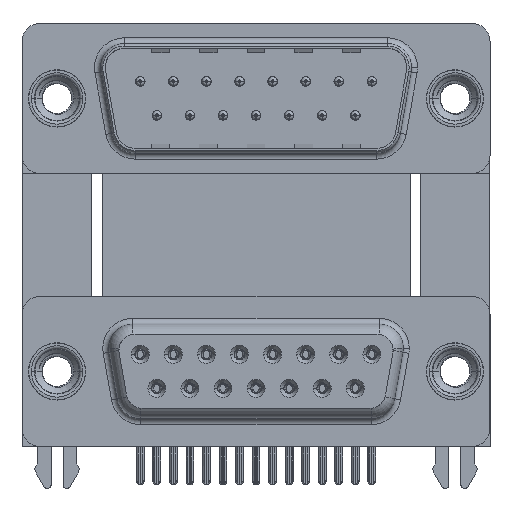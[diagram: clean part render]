
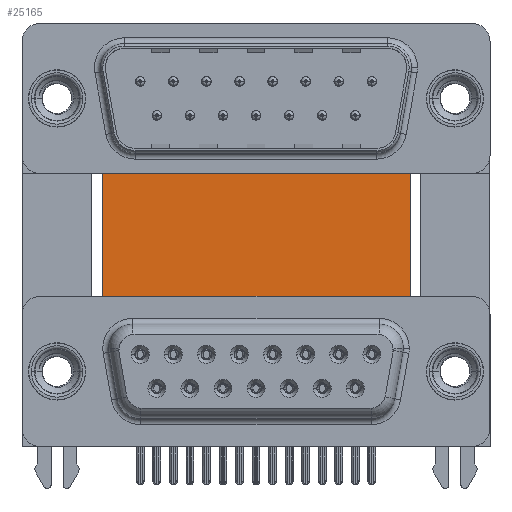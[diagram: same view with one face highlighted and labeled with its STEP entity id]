
A CAD part, top view. The second image highlights one B-rep face of the part: STEP entity #25165.
In plain terms, the highlighted planar face has unit normal (0, 0, 1).
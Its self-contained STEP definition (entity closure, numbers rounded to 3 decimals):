
#782 = CARTESIAN_POINT ( 'NONE',  ( 3.79, 16.585, -12. ) ) ;
#2208 = EDGE_CURVE ( 'NONE', #26414, #30153, #3632, .T. ) ;
#3604 = VECTOR ( 'NONE', #38232, 1000. ) ;
#3632 = LINE ( 'NONE', #45953, #9818 ) ;
#8812 = PLANE ( 'NONE',  #43864 ) ;
#9621 = ORIENTED_EDGE ( 'NONE', *, *, #45818, .T. ) ;
#9818 = VECTOR ( 'NONE', #28023, 1000. ) ;
#10220 = CARTESIAN_POINT ( 'NONE',  ( 29.58, 16.585, -12. ) ) ;
#11406 = VECTOR ( 'NONE', #35370, 1000. ) ;
#13543 = ORIENTED_EDGE ( 'NONE', *, *, #38577, .F. ) ;
#17365 = DIRECTION ( 'NONE',  ( 1., 0., 0. ) ) ;
#17834 = CARTESIAN_POINT ( 'NONE',  ( 3.79, -3.735, -12. ) ) ;
#18302 = CARTESIAN_POINT ( 'NONE',  ( 3.79, -3.735, -12. ) ) ;
#19711 = DIRECTION ( 'NONE',  ( 0., 0., -1. ) ) ;
#19946 = CARTESIAN_POINT ( 'NONE',  ( 3.79, 16.585, -12. ) ) ;
#21099 = LINE ( 'NONE', #17834, #30409 ) ;
#23047 = EDGE_CURVE ( 'NONE', #38837, #30054, #35429, .T. ) ;
#23661 = DIRECTION ( 'NONE',  ( -1., 0., 0. ) ) ;
#25165 = ADVANCED_FACE ( 'NONE', ( #37156 ), #8812, .F. ) ;
#26414 = VERTEX_POINT ( 'NONE', #10220 ) ;
#27279 = EDGE_LOOP ( 'NONE', ( #9621, #29055, #13543, #40068 ) ) ;
#28023 = DIRECTION ( 'NONE',  ( 0., -1., 0. ) ) ;
#29055 = ORIENTED_EDGE ( 'NONE', *, *, #2208, .F. ) ;
#30054 = VERTEX_POINT ( 'NONE', #18302 ) ;
#30153 = VERTEX_POINT ( 'NONE', #35458 ) ;
#30409 = VECTOR ( 'NONE', #17365, 1000. ) ;
#32186 = CARTESIAN_POINT ( 'NONE',  ( 3.79, 16.585, -12. ) ) ;
#35370 = DIRECTION ( 'NONE',  ( 1., 0., 0. ) ) ;
#35429 = LINE ( 'NONE', #32186, #3604 ) ;
#35458 = CARTESIAN_POINT ( 'NONE',  ( 29.58, -3.735, -12. ) ) ;
#36052 = LINE ( 'NONE', #38870, #11406 ) ;
#37156 = FACE_OUTER_BOUND ( 'NONE', #27279, .T. ) ;
#38232 = DIRECTION ( 'NONE',  ( 0., -1., 0. ) ) ;
#38577 = EDGE_CURVE ( 'NONE', #38837, #26414, #36052, .T. ) ;
#38837 = VERTEX_POINT ( 'NONE', #782 ) ;
#38870 = CARTESIAN_POINT ( 'NONE',  ( 3.79, 16.585, -12. ) ) ;
#40068 = ORIENTED_EDGE ( 'NONE', *, *, #23047, .T. ) ;
#43864 = AXIS2_PLACEMENT_3D ( 'NONE', #19946, #19711, #23661 ) ;
#45818 = EDGE_CURVE ( 'NONE', #30054, #30153, #21099, .T. ) ;
#45953 = CARTESIAN_POINT ( 'NONE',  ( 29.58, 16.585, -12. ) ) ;
